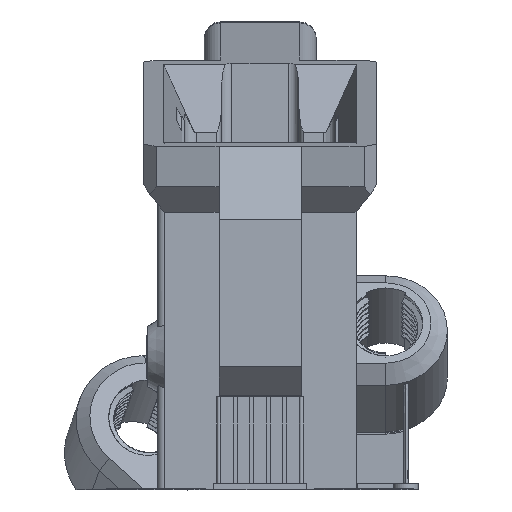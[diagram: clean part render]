
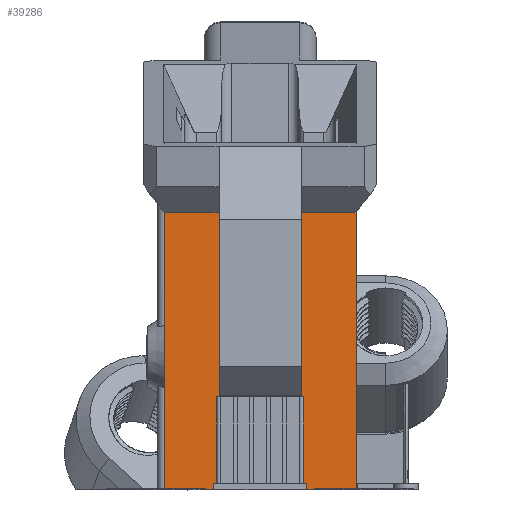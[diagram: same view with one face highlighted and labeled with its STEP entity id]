
A CAD part, left-side view. The second image highlights one B-rep face of the part: STEP entity #39286.
In plain terms, the highlighted planar face has unit normal (-1, 0, 0).
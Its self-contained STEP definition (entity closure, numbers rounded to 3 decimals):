
#1803=PLANE('',#41097);
#3576=FACE_OUTER_BOUND('',#5775,.T.);
#5775=EDGE_LOOP('',(#30748,#30749,#30750,#30751,#30752,#30753,#30754,#30755,
#30756,#30757,#30758,#30759));
#10530=LINE('',#61278,#14101);
#10537=LINE('',#61338,#14108);
#10538=LINE('',#61340,#14109);
#10539=LINE('',#61342,#14110);
#10540=LINE('',#61344,#14111);
#10541=LINE('',#61346,#14112);
#10542=LINE('',#61348,#14113);
#10543=LINE('',#61350,#14114);
#10544=LINE('',#61352,#14115);
#10545=LINE('',#61354,#14116);
#10546=LINE('',#61356,#14117);
#10547=LINE('',#61357,#14118);
#14101=VECTOR('',#44569,1000.);
#14108=VECTOR('',#44588,1000.);
#14109=VECTOR('',#44589,1000.);
#14110=VECTOR('',#44590,1000.);
#14111=VECTOR('',#44591,1000.);
#14112=VECTOR('',#44592,1000.);
#14113=VECTOR('',#44593,1000.);
#14114=VECTOR('',#44594,1000.);
#14115=VECTOR('',#44595,1000.);
#14116=VECTOR('',#44596,1000.);
#14117=VECTOR('',#44597,1000.);
#14118=VECTOR('',#44598,1000.);
#17848=VERTEX_POINT('',#61275);
#17849=VERTEX_POINT('',#61277);
#17860=VERTEX_POINT('',#61337);
#17861=VERTEX_POINT('',#61339);
#17862=VERTEX_POINT('',#61341);
#17863=VERTEX_POINT('',#61343);
#17864=VERTEX_POINT('',#61345);
#17865=VERTEX_POINT('',#61347);
#17866=VERTEX_POINT('',#61349);
#17867=VERTEX_POINT('',#61351);
#17868=VERTEX_POINT('',#61353);
#17869=VERTEX_POINT('',#61355);
#22581=EDGE_CURVE('',#17848,#17849,#10530,.T.);
#22595=EDGE_CURVE('',#17848,#17860,#10537,.T.);
#22596=EDGE_CURVE('',#17860,#17861,#10538,.T.);
#22597=EDGE_CURVE('',#17862,#17861,#10539,.T.);
#22598=EDGE_CURVE('',#17863,#17862,#10540,.T.);
#22599=EDGE_CURVE('',#17863,#17864,#10541,.T.);
#22600=EDGE_CURVE('',#17864,#17865,#10542,.T.);
#22601=EDGE_CURVE('',#17865,#17866,#10543,.T.);
#22602=EDGE_CURVE('',#17866,#17867,#10544,.T.);
#22603=EDGE_CURVE('',#17867,#17868,#10545,.T.);
#22604=EDGE_CURVE('',#17869,#17868,#10546,.T.);
#22605=EDGE_CURVE('',#17869,#17849,#10547,.T.);
#30748=ORIENTED_EDGE('',*,*,#22581,.F.);
#30749=ORIENTED_EDGE('',*,*,#22595,.T.);
#30750=ORIENTED_EDGE('',*,*,#22596,.T.);
#30751=ORIENTED_EDGE('',*,*,#22597,.F.);
#30752=ORIENTED_EDGE('',*,*,#22598,.F.);
#30753=ORIENTED_EDGE('',*,*,#22599,.T.);
#30754=ORIENTED_EDGE('',*,*,#22600,.T.);
#30755=ORIENTED_EDGE('',*,*,#22601,.T.);
#30756=ORIENTED_EDGE('',*,*,#22602,.T.);
#30757=ORIENTED_EDGE('',*,*,#22603,.T.);
#30758=ORIENTED_EDGE('',*,*,#22604,.F.);
#30759=ORIENTED_EDGE('',*,*,#22605,.T.);
#39286=ADVANCED_FACE('',(#3576),#1803,.F.);
#41097=AXIS2_PLACEMENT_3D('',#61336,#44586,#44587);
#44569=DIRECTION('',(0.,0.,-1.));
#44586=DIRECTION('center_axis',(1.,0.,0.));
#44587=DIRECTION('ref_axis',(0.,1.,0.));
#44588=DIRECTION('',(0.,1.,0.));
#44589=DIRECTION('',(0.,0.,-1.));
#44590=DIRECTION('',(0.,-1.,0.));
#44591=DIRECTION('',(0.,0.,-1.));
#44592=DIRECTION('',(0.,1.,0.));
#44593=DIRECTION('',(0.,0.,-1.));
#44594=DIRECTION('',(0.,-1.,0.));
#44595=DIRECTION('',(0.,0.,-1.));
#44596=DIRECTION('',(0.,-1.,0.));
#44597=DIRECTION('',(0.,0.,-1.));
#44598=DIRECTION('',(0.,-1.,0.));
#61275=CARTESIAN_POINT('',(-90.475,9.53,63.957));
#61277=CARTESIAN_POINT('',(-90.475,9.53,21.237));
#61278=CARTESIAN_POINT('',(-90.475,9.53,46.437));
#61336=CARTESIAN_POINT('Origin',(-90.475,17.988,46.437));
#61337=CARTESIAN_POINT('',(-90.475,17.988,63.957));
#61338=CARTESIAN_POINT('',(-90.475,-2.332,63.957));
#61339=CARTESIAN_POINT('',(-90.475,17.988,35.642));
#61340=CARTESIAN_POINT('',(-90.475,17.988,63.957));
#61341=CARTESIAN_POINT('',(-90.475,30.688,35.642));
#61342=CARTESIAN_POINT('',(-90.475,63.789,35.642));
#61343=CARTESIAN_POINT('',(-90.475,30.688,63.957));
#61344=CARTESIAN_POINT('',(-90.475,30.688,21.037));
#61345=CARTESIAN_POINT('',(-90.475,39.146,63.957));
#61346=CARTESIAN_POINT('',(-90.475,-2.332,63.957));
#61347=CARTESIAN_POINT('',(-90.475,39.146,21.237));
#61348=CARTESIAN_POINT('',(-90.475,39.146,46.437));
#61349=CARTESIAN_POINT('',(-90.475,32.796,21.237));
#61350=CARTESIAN_POINT('',(-90.475,32.796,21.237));
#61351=CARTESIAN_POINT('',(-90.475,32.796,21.037));
#61352=CARTESIAN_POINT('',(-90.475,32.796,21.237));
#61353=CARTESIAN_POINT('',(-90.475,15.88,21.037));
#61354=CARTESIAN_POINT('',(-90.475,17.988,21.037));
#61355=CARTESIAN_POINT('',(-90.475,15.88,21.237));
#61356=CARTESIAN_POINT('',(-90.475,15.88,21.237));
#61357=CARTESIAN_POINT('',(-90.475,15.88,21.237));
